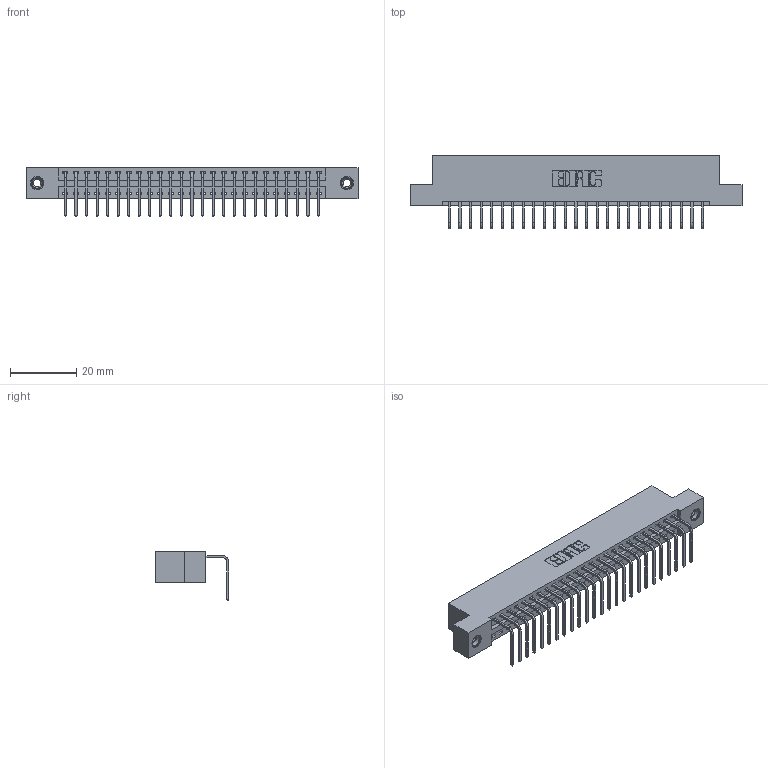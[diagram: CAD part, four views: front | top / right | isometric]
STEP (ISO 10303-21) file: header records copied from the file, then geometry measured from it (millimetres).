
FILE_DESCRIPTION (( 'STEP AP203' ), '1' );
FILE_NAME ('396-025-558-108.STEP', '2019-11-01T06:31:05', ( '' ), ( '' ), 'SwSTEP 2.0', 'SolidWorks 2016', '' );
FILE_SCHEMA (( 'CONFIG_CONTROL_DESIGN' ));
Length unit declared in the file: inch
Products named in the file (4): 346 Part_Flush Mounting Lugs - 0.156 Dia-TI; 345-292-001_558 Tail - 2; 345-250-001_345-250-003-102; 396-025-558-108
Assembly tree (28 placements, depth 2):
  396-025-558-108
    346 Part_Flush Mounting Lugs - 0.156 Dia-TI
    345-292-001_558 Tail - 2  x25
    345-250-001_345-250-003-102  x2
Bounding box: 99.95 x 22.16 x 14.73 mm (x, y, z)
Volume: 9527 mm3; surface area: 12242.8 mm2
Topology: 28 solids, 28 shells, 1682 faces, 5015 edges, 3302 vertices
Faces by surface type: plane 1158, cylinder 508, cone 12, torus 4
Entity records: 19074 total; most frequent: CARTESIAN_POINT 3258, ORIENTED_EDGE 3210, DIRECTION 2921, EDGE_CURVE 1605, VECTOR 1353, LINE 1353, VERTEX_POINT 1064, AXIS2_PLACEMENT_3D 784
